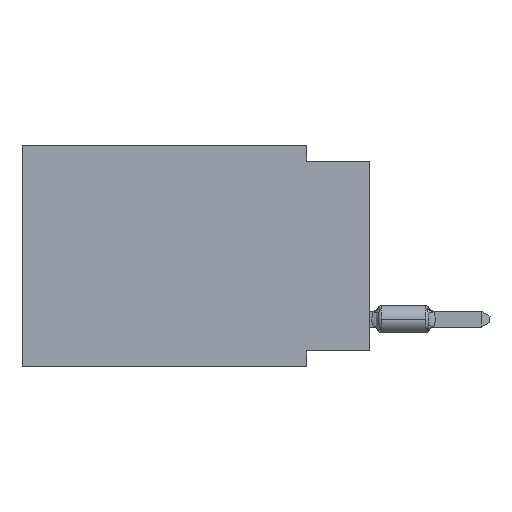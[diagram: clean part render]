
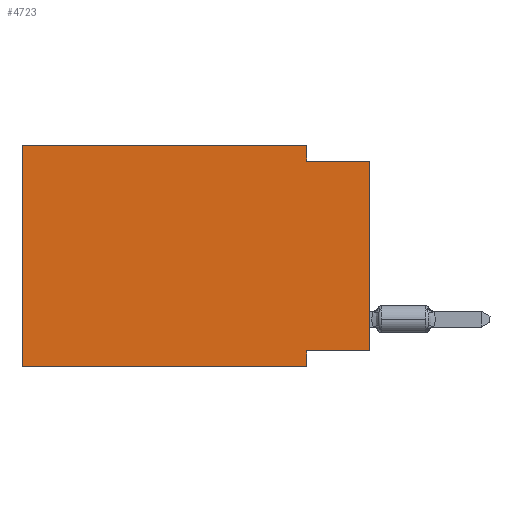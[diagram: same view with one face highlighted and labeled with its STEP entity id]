
A CAD part, left-side view. The second image highlights one B-rep face of the part: STEP entity #4723.
In plain terms, the highlighted planar face has unit normal (-1, 0, 0).
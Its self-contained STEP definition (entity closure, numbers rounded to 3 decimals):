
#177 = DIRECTION ( 'NONE',  ( 0., 0., 1. ) ) ;
#1068 = LINE ( 'NONE', #4322, #11937 ) ;
#1568 = CARTESIAN_POINT ( 'NONE',  ( 0., 0., 0. ) ) ;
#1786 = EDGE_LOOP ( 'NONE', ( #18208, #4165, #4276, #12014, #13007, #10558, #2791, #2730 ) ) ;
#2503 = CARTESIAN_POINT ( 'NONE',  ( 0., 2.54, -8.89 ) ) ;
#2730 = ORIENTED_EDGE ( 'NONE', *, *, #14349, .F. ) ;
#2791 = ORIENTED_EDGE ( 'NONE', *, *, #17550, .F. ) ;
#3183 = VECTOR ( 'NONE', #8408, 1000. ) ;
#3654 = DIRECTION ( 'NONE',  ( 0., 0., -1. ) ) ;
#4019 = VECTOR ( 'NONE', #3654, 1000. ) ;
#4093 = DIRECTION ( 'NONE',  ( 0., -1., 0. ) ) ;
#4165 = ORIENTED_EDGE ( 'NONE', *, *, #10532, .F. ) ;
#4276 = ORIENTED_EDGE ( 'NONE', *, *, #13652, .F. ) ;
#4322 = CARTESIAN_POINT ( 'NONE',  ( 0., 0., -8.255 ) ) ;
#4626 = VECTOR ( 'NONE', #4093, 1000. ) ;
#4689 = CARTESIAN_POINT ( 'NONE',  ( 0., 13.97, 0. ) ) ;
#4723 = ADVANCED_FACE ( 'NONE', ( #6156 ), #15342, .F. ) ;
#5184 = EDGE_CURVE ( 'NONE', #18672, #18307, #15759, .T. ) ;
#5533 = VECTOR ( 'NONE', #11474, 1000. ) ;
#5838 = LINE ( 'NONE', #17567, #9027 ) ;
#6156 = FACE_OUTER_BOUND ( 'NONE', #1786, .T. ) ;
#6260 = DIRECTION ( 'NONE',  ( 0., 0., -1. ) ) ;
#6728 = CARTESIAN_POINT ( 'NONE',  ( 0., 2.54, 0. ) ) ;
#7382 = AXIS2_PLACEMENT_3D ( 'NONE', #4689, #12120, #6260 ) ;
#7390 = VECTOR ( 'NONE', #17324, 1000. ) ;
#8408 = DIRECTION ( 'NONE',  ( 0., 0., -1. ) ) ;
#8453 = CARTESIAN_POINT ( 'NONE',  ( 0., 13.97, 0. ) ) ;
#8728 = DIRECTION ( 'NONE',  ( 0., 1., 0. ) ) ;
#9027 = VECTOR ( 'NONE', #16480, 1000. ) ;
#9044 = VECTOR ( 'NONE', #177, 1000. ) ;
#9454 = CARTESIAN_POINT ( 'NONE',  ( 0., 2.54, -8.255 ) ) ;
#9775 = CARTESIAN_POINT ( 'NONE',  ( 0., 2.54, 0. ) ) ;
#9857 = LINE ( 'NONE', #14167, #4626 ) ;
#10532 = EDGE_CURVE ( 'NONE', #12705, #14615, #17634, .T. ) ;
#10558 = ORIENTED_EDGE ( 'NONE', *, *, #17216, .T. ) ;
#11321 = EDGE_CURVE ( 'NONE', #18307, #11395, #9857, .T. ) ;
#11395 = VERTEX_POINT ( 'NONE', #6728 ) ;
#11474 = DIRECTION ( 'NONE',  ( 0., -1., 0. ) ) ;
#11937 = VECTOR ( 'NONE', #8728, 1000. ) ;
#12014 = ORIENTED_EDGE ( 'NONE', *, *, #11321, .F. ) ;
#12120 = DIRECTION ( 'NONE',  ( 1., 0., 0. ) ) ;
#12332 = EDGE_CURVE ( 'NONE', #15451, #14615, #14971, .T. ) ;
#12705 = VERTEX_POINT ( 'NONE', #16604 ) ;
#13007 = ORIENTED_EDGE ( 'NONE', *, *, #5184, .F. ) ;
#13145 = CARTESIAN_POINT ( 'NONE',  ( 0., 0., -0.635 ) ) ;
#13652 = EDGE_CURVE ( 'NONE', #11395, #12705, #17284, .T. ) ;
#14167 = CARTESIAN_POINT ( 'NONE',  ( 0., 13.97, 0. ) ) ;
#14349 = EDGE_CURVE ( 'NONE', #15451, #17373, #1068, .T. ) ;
#14424 = CARTESIAN_POINT ( 'NONE',  ( 0., 2.54, -8.89 ) ) ;
#14615 = VERTEX_POINT ( 'NONE', #18655 ) ;
#14971 = LINE ( 'NONE', #1568, #9044 ) ;
#15342 = PLANE ( 'NONE',  #7382 ) ;
#15451 = VERTEX_POINT ( 'NONE', #18704 ) ;
#15759 = LINE ( 'NONE', #8453, #7390 ) ;
#16350 = VERTEX_POINT ( 'NONE', #2503 ) ;
#16480 = DIRECTION ( 'NONE',  ( 0., -1., 0. ) ) ;
#16604 = CARTESIAN_POINT ( 'NONE',  ( 0., 2.54, -0.635 ) ) ;
#17039 = LINE ( 'NONE', #14424, #4019 ) ;
#17092 = CARTESIAN_POINT ( 'NONE',  ( 0., 13.97, 0. ) ) ;
#17216 = EDGE_CURVE ( 'NONE', #18672, #16350, #5838, .T. ) ;
#17284 = LINE ( 'NONE', #9775, #3183 ) ;
#17324 = DIRECTION ( 'NONE',  ( 0., 0., 1. ) ) ;
#17373 = VERTEX_POINT ( 'NONE', #9454 ) ;
#17550 = EDGE_CURVE ( 'NONE', #17373, #16350, #17039, .T. ) ;
#17567 = CARTESIAN_POINT ( 'NONE',  ( 0., 13.97, -8.89 ) ) ;
#17634 = LINE ( 'NONE', #13145, #5533 ) ;
#18208 = ORIENTED_EDGE ( 'NONE', *, *, #12332, .T. ) ;
#18307 = VERTEX_POINT ( 'NONE', #17092 ) ;
#18450 = CARTESIAN_POINT ( 'NONE',  ( 0., 13.97, -8.89 ) ) ;
#18655 = CARTESIAN_POINT ( 'NONE',  ( 0., 0., -0.635 ) ) ;
#18672 = VERTEX_POINT ( 'NONE', #18450 ) ;
#18704 = CARTESIAN_POINT ( 'NONE',  ( 0., 0., -8.255 ) ) ;
